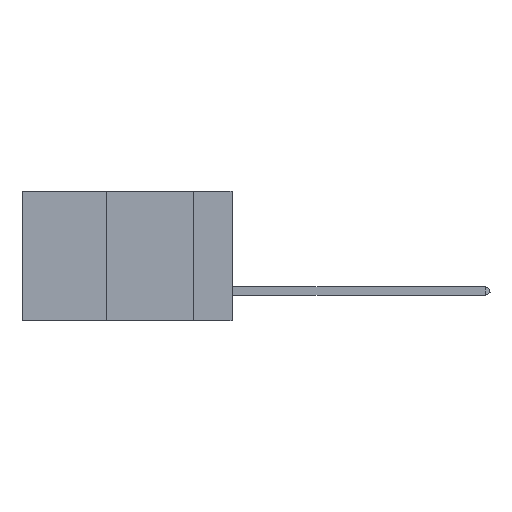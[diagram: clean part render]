
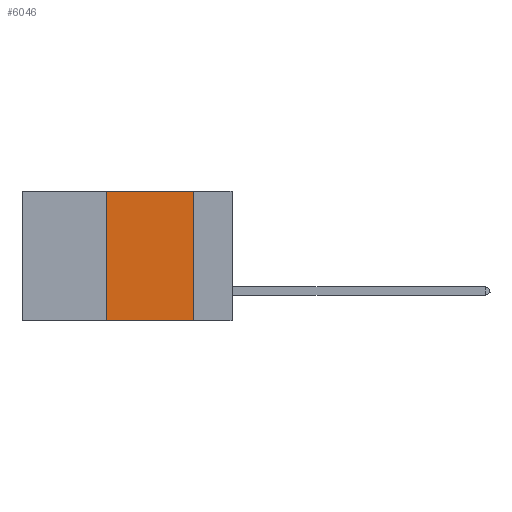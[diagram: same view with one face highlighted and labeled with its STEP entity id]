
A CAD part, left-side view. The second image highlights one B-rep face of the part: STEP entity #6046.
In plain terms, the highlighted planar face has unit normal (-1, 0, 0).
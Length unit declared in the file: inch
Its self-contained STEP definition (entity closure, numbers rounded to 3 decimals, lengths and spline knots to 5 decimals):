
#535 = ORIENTED_EDGE ( 'NONE', *, *, #32445, .F. ) ;
#1106 = VERTEX_POINT ( 'NONE', #24163 ) ;
#2301 = EDGE_CURVE ( 'NONE', #23965, #6285, #39252, .T. ) ;
#2961 = EDGE_CURVE ( 'NONE', #1106, #11626, #3756, .T. ) ;
#3604 = DIRECTION ( 'NONE',  ( 0., -1., 0. ) ) ;
#3756 = LINE ( 'NONE', #19081, #8763 ) ;
#4795 = ORIENTED_EDGE ( 'NONE', *, *, #28559, .F. ) ;
#6046 = ADVANCED_FACE ( 'NONE', ( #16300 ), #15621, .F. ) ;
#6285 = VERTEX_POINT ( 'NONE', #38620 ) ;
#6403 = CARTESIAN_POINT ( 'NONE',  ( 0., 0.36, 0. ) ) ;
#7648 = VECTOR ( 'NONE', #22334, 39.37008 ) ;
#8347 = VECTOR ( 'NONE', #10055, 39.37008 ) ;
#8763 = VECTOR ( 'NONE', #3604, 39.37008 ) ;
#10055 = DIRECTION ( 'NONE',  ( 0., 0., -1. ) ) ;
#11626 = VERTEX_POINT ( 'NONE', #14551 ) ;
#13060 = CARTESIAN_POINT ( 'NONE',  ( 0., 0.11, 0. ) ) ;
#14551 = CARTESIAN_POINT ( 'NONE',  ( 0., 0.11, -0.37 ) ) ;
#15621 = PLANE ( 'NONE',  #17311 ) ;
#16300 = FACE_OUTER_BOUND ( 'NONE', #40531, .T. ) ;
#16654 = CARTESIAN_POINT ( 'NONE',  ( 0., 0.6, 0. ) ) ;
#17311 = AXIS2_PLACEMENT_3D ( 'NONE', #16654, #26357, #20558 ) ;
#19081 = CARTESIAN_POINT ( 'NONE',  ( 0., 0.6, -0.37 ) ) ;
#20558 = DIRECTION ( 'NONE',  ( 0., 0., -1. ) ) ;
#21655 = LINE ( 'NONE', #13060, #8347 ) ;
#21986 = DIRECTION ( 'NONE',  ( 0., 0., 1. ) ) ;
#22334 = DIRECTION ( 'NONE',  ( 0., -1., 0. ) ) ;
#22461 = LINE ( 'NONE', #6403, #33328 ) ;
#23965 = VERTEX_POINT ( 'NONE', #35188 ) ;
#24163 = CARTESIAN_POINT ( 'NONE',  ( 0., 0.36, -0.37 ) ) ;
#26357 = DIRECTION ( 'NONE',  ( 1., 0., 0. ) ) ;
#27666 = ORIENTED_EDGE ( 'NONE', *, *, #2301, .F. ) ;
#28559 = EDGE_CURVE ( 'NONE', #1106, #23965, #22461, .T. ) ;
#32263 = CARTESIAN_POINT ( 'NONE',  ( 0., 0.6, 0. ) ) ;
#32445 = EDGE_CURVE ( 'NONE', #6285, #11626, #21655, .T. ) ;
#33328 = VECTOR ( 'NONE', #21986, 39.37008 ) ;
#35188 = CARTESIAN_POINT ( 'NONE',  ( 0., 0.36, 0. ) ) ;
#37772 = ORIENTED_EDGE ( 'NONE', *, *, #2961, .T. ) ;
#38620 = CARTESIAN_POINT ( 'NONE',  ( 0., 0.11, 0. ) ) ;
#39252 = LINE ( 'NONE', #32263, #7648 ) ;
#40531 = EDGE_LOOP ( 'NONE', ( #535, #27666, #4795, #37772 ) ) ;
